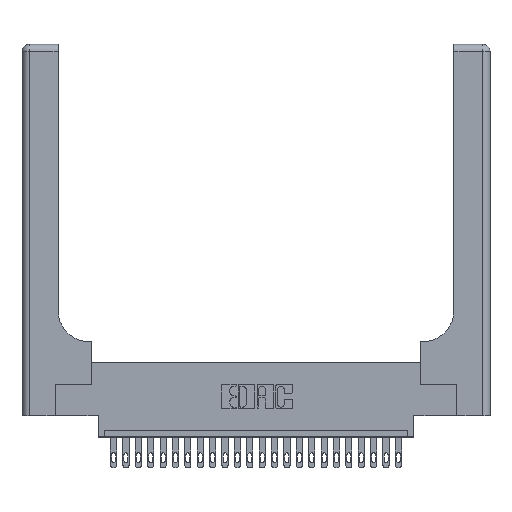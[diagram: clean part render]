
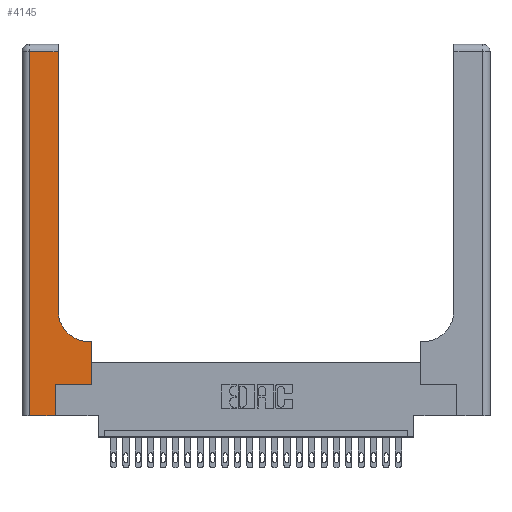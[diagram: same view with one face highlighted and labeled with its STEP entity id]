
A CAD part, top view. The second image highlights one B-rep face of the part: STEP entity #4145.
In plain terms, the highlighted planar face has unit normal (0, 0, 1).
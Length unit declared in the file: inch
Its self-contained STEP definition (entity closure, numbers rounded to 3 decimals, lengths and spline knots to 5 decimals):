
#126 = AXIS2_PLACEMENT_3D ( 'NONE', #14502, #20532, #20450 ) ;
#168 = ORIENTED_EDGE ( 'NONE', *, *, #5739, .T. ) ;
#338 = ORIENTED_EDGE ( 'NONE', *, *, #17445, .T. ) ;
#356 = ORIENTED_EDGE ( 'NONE', *, *, #13082, .T. ) ;
#522 = VERTEX_POINT ( 'NONE', #7391 ) ;
#1535 = VECTOR ( 'NONE', #19175, 39.37008 ) ;
#1654 = ORIENTED_EDGE ( 'NONE', *, *, #4995, .T. ) ;
#1707 = CARTESIAN_POINT ( 'NONE',  ( 0.5585, 0.6, 0.37 ) ) ;
#2416 = CARTESIAN_POINT ( 'NONE',  ( 0., 2.94, 0.37 ) ) ;
#2592 = ORIENTED_EDGE ( 'NONE', *, *, #17301, .T. ) ;
#3163 = CARTESIAN_POINT ( 'NONE',  ( 0.5585, 0.25, 0.37 ) ) ;
#3812 = DIRECTION ( 'NONE',  ( 0., 1., 0. ) ) ;
#4145 = ADVANCED_FACE ( 'NONE', ( #17537 ), #12377, .F. ) ;
#4418 = CIRCLE ( 'NONE', #126, 0.25 ) ;
#4910 = LINE ( 'NONE', #18365, #12054 ) ;
#4995 = EDGE_CURVE ( 'NONE', #7395, #10505, #4418, .T. ) ;
#5257 = CARTESIAN_POINT ( 'NONE',  ( 0., 0., 0.37 ) ) ;
#5739 = EDGE_CURVE ( 'NONE', #23093, #18315, #10581, .T. ) ;
#6160 = LINE ( 'NONE', #18801, #17671 ) ;
#6567 = DIRECTION ( 'NONE',  ( 0., 1., 0. ) ) ;
#6829 = VECTOR ( 'NONE', #3812, 39.37008 ) ;
#7165 = ORIENTED_EDGE ( 'NONE', *, *, #9355, .T. ) ;
#7391 = CARTESIAN_POINT ( 'NONE',  ( 0.269, 0., 0.37 ) ) ;
#7395 = VERTEX_POINT ( 'NONE', #22392 ) ;
#7877 = LINE ( 'NONE', #2416, #9442 ) ;
#8055 = CARTESIAN_POINT ( 'NONE',  ( 0.2915, 0.85, 0.37 ) ) ;
#8081 = VERTEX_POINT ( 'NONE', #21706 ) ;
#8879 = ORIENTED_EDGE ( 'NONE', *, *, #24033, .T. ) ;
#9355 = EDGE_CURVE ( 'NONE', #8081, #522, #20530, .T. ) ;
#9442 = VECTOR ( 'NONE', #18340, 39.37008 ) ;
#10287 = ORIENTED_EDGE ( 'NONE', *, *, #10515, .T. ) ;
#10505 = VERTEX_POINT ( 'NONE', #8055 ) ;
#10515 = EDGE_CURVE ( 'NONE', #18315, #7395, #20461, .T. ) ;
#10581 = LINE ( 'NONE', #3163, #24233 ) ;
#10647 = CARTESIAN_POINT ( 'NONE',  ( 0., 3., 0.37 ) ) ;
#11528 = VERTEX_POINT ( 'NONE', #13327 ) ;
#11997 = LINE ( 'NONE', #23844, #22838 ) ;
#12054 = VECTOR ( 'NONE', #22084, 39.37008 ) ;
#12377 = PLANE ( 'NONE',  #18127 ) ;
#12841 = CARTESIAN_POINT ( 'NONE',  ( 0.06, 2.94, 0.37 ) ) ;
#13082 = EDGE_CURVE ( 'NONE', #11528, #24427, #7877, .T. ) ;
#13327 = CARTESIAN_POINT ( 'NONE',  ( 0.2915, 2.94, 0.37 ) ) ;
#14046 = CARTESIAN_POINT ( 'NONE',  ( 0.2915, 3., 0.37 ) ) ;
#14277 = DIRECTION ( 'NONE',  ( 0., 0., -1. ) ) ;
#14502 = CARTESIAN_POINT ( 'NONE',  ( 0.5415, 0.85, 0.37 ) ) ;
#16273 = CARTESIAN_POINT ( 'NONE',  ( 0.269, 0.25, 0.37 ) ) ;
#16330 = ORIENTED_EDGE ( 'NONE', *, *, #18853, .T. ) ;
#16402 = CARTESIAN_POINT ( 'NONE',  ( 0.5585, 0.25, 0.37 ) ) ;
#17301 = EDGE_CURVE ( 'NONE', #19491, #23093, #4910, .T. ) ;
#17445 = EDGE_CURVE ( 'NONE', #24427, #8081, #6160, .T. ) ;
#17537 = FACE_OUTER_BOUND ( 'NONE', #17991, .T. ) ;
#17671 = VECTOR ( 'NONE', #20894, 39.37008 ) ;
#17991 = EDGE_LOOP ( 'NONE', ( #8879, #356, #338, #7165, #16330, #2592, #168, #10287, #1654 ) ) ;
#18127 = AXIS2_PLACEMENT_3D ( 'NONE', #10647, #14277, #18380 ) ;
#18315 = VERTEX_POINT ( 'NONE', #1707 ) ;
#18340 = DIRECTION ( 'NONE',  ( -1., 0., 0. ) ) ;
#18365 = CARTESIAN_POINT ( 'NONE',  ( 0.269, 0.25, 0.37 ) ) ;
#18380 = DIRECTION ( 'NONE',  ( -1., 0., 0. ) ) ;
#18801 = CARTESIAN_POINT ( 'NONE',  ( 0.06, 3., 0.37 ) ) ;
#18853 = EDGE_CURVE ( 'NONE', #522, #19491, #11997, .T. ) ;
#19175 = DIRECTION ( 'NONE',  ( 1., 0., 0. ) ) ;
#19491 = VERTEX_POINT ( 'NONE', #16273 ) ;
#20008 = CARTESIAN_POINT ( 'NONE',  ( 0.2915, 0.6, 0.37 ) ) ;
#20450 = DIRECTION ( 'NONE',  ( 1., 0., 0. ) ) ;
#20461 = LINE ( 'NONE', #20008, #21693 ) ;
#20530 = LINE ( 'NONE', #5257, #1535 ) ;
#20532 = DIRECTION ( 'NONE',  ( 0., 0., -1. ) ) ;
#20590 = DIRECTION ( 'NONE',  ( -1., 0., 0. ) ) ;
#20894 = DIRECTION ( 'NONE',  ( 0., -1., 0. ) ) ;
#21081 = DIRECTION ( 'NONE',  ( 0., 1., 0. ) ) ;
#21693 = VECTOR ( 'NONE', #20590, 39.37008 ) ;
#21706 = CARTESIAN_POINT ( 'NONE',  ( 0.06, 0., 0.37 ) ) ;
#22084 = DIRECTION ( 'NONE',  ( 1., 0., 0. ) ) ;
#22392 = CARTESIAN_POINT ( 'NONE',  ( 0.5415, 0.6, 0.37 ) ) ;
#22838 = VECTOR ( 'NONE', #6567, 39.37008 ) ;
#23093 = VERTEX_POINT ( 'NONE', #16402 ) ;
#23277 = LINE ( 'NONE', #14046, #6829 ) ;
#23844 = CARTESIAN_POINT ( 'NONE',  ( 0.269, 0., 0.37 ) ) ;
#24033 = EDGE_CURVE ( 'NONE', #10505, #11528, #23277, .T. ) ;
#24233 = VECTOR ( 'NONE', #21081, 39.37008 ) ;
#24427 = VERTEX_POINT ( 'NONE', #12841 ) ;
